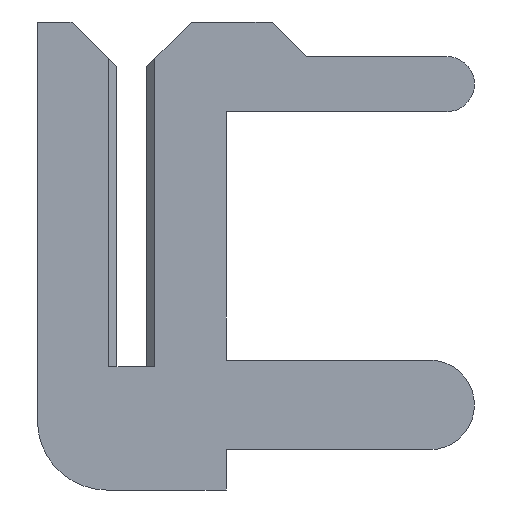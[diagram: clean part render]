
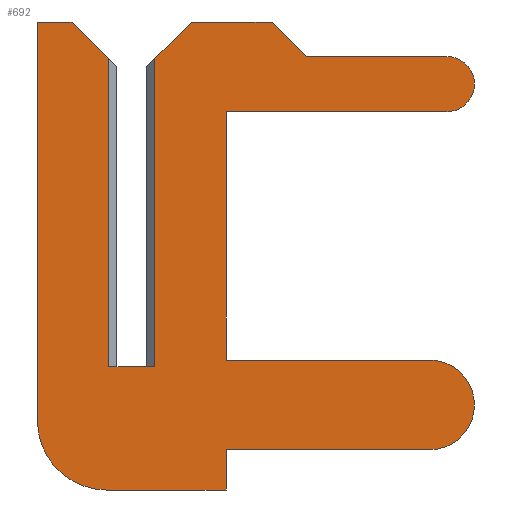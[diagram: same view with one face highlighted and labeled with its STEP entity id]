
A CAD part, left-side view. The second image highlights one B-rep face of the part: STEP entity #692.
In plain terms, the highlighted planar face has unit normal (-1, 0, 0).
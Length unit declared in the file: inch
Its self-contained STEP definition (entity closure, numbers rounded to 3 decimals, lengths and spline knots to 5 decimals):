
#9 = VECTOR ( 'NONE', #65, 39.37008 ) ;
#14 = DIRECTION ( 'NONE',  ( 0., 0., 1. ) ) ;
#15 = CARTESIAN_POINT ( 'NONE',  ( -0.01, -0.01, 0.134 ) ) ;
#26 = EDGE_CURVE ( 'NONE', #310, #512, #950, .T. ) ;
#29 = DIRECTION ( 'NONE',  ( 0., 0., -1. ) ) ;
#35 = CARTESIAN_POINT ( 'NONE',  ( -0.01, -0.076, 0.135 ) ) ;
#43 = VERTEX_POINT ( 'NONE', #170 ) ;
#44 = EDGE_CURVE ( 'NONE', #637, #543, #290, .T. ) ;
#54 = AXIS2_PLACEMENT_3D ( 'NONE', #1008, #584, #843 ) ;
#57 = CIRCLE ( 'NONE', #408, 0.0195 ) ;
#65 = DIRECTION ( 'NONE',  ( 0., 1., 0. ) ) ;
#67 = VERTEX_POINT ( 'NONE', #343 ) ;
#74 = AXIS2_PLACEMENT_3D ( 'NONE', #490, #242, #400 ) ;
#76 = VERTEX_POINT ( 'NONE', #622 ) ;
#88 = VECTOR ( 'NONE', #841, 39.37008 ) ;
#93 = CARTESIAN_POINT ( 'NONE',  ( -0.01, 0.026, 0.15 ) ) ;
#95 = CARTESIAN_POINT ( 'NONE',  ( -0.01, -0.1295, 0.003 ) ) ;
#98 = CARTESIAN_POINT ( 'NONE',  ( -0.01, 0.011, -0.0235 ) ) ;
#99 = LINE ( 'NONE', #196, #718 ) ;
#103 = EDGE_CURVE ( 'NONE', #399, #998, #57, .T. ) ;
#108 = CARTESIAN_POINT ( 'NONE',  ( -0.01, 0.041, 0.15 ) ) ;
#115 = VERTEX_POINT ( 'NONE', #700 ) ;
#123 = DIRECTION ( 'NONE',  ( 0., 0., 1. ) ) ;
#134 = EDGE_CURVE ( 'NONE', #356, #43, #860, .T. ) ;
#135 = LINE ( 'NONE', #108, #788 ) ;
#137 = DIRECTION ( 'NONE',  ( 0., 0., -1. ) ) ;
#145 = ORIENTED_EDGE ( 'NONE', *, *, #157, .F. ) ;
#155 = CARTESIAN_POINT ( 'NONE',  ( -0.01, -0.137, 0.135 ) ) ;
#157 = EDGE_CURVE ( 'NONE', #619, #431, #603, .T. ) ;
#170 = CARTESIAN_POINT ( 'NONE',  ( -0.01, -0.01, 0. ) ) ;
#180 = DIRECTION ( 'NONE',  ( 0., 1., 0. ) ) ;
#191 = LINE ( 'NONE', #1004, #9 ) ;
#195 = DIRECTION ( 'NONE',  ( 0., 1., 0. ) ) ;
#196 = CARTESIAN_POINT ( 'NONE',  ( -0.01, 0.01, -0.0235 ) ) ;
#198 = EDGE_LOOP ( 'NONE', ( #536, #684, #550, #1042, #621, #262, #651, #298, #620, #1079, #559, #703, #541, #442, #145, #604, #933, #417, #813 ) ) ;
#203 = CARTESIAN_POINT ( 'NONE',  ( -0.01, -0.076, 0.135 ) ) ;
#212 = CARTESIAN_POINT ( 'NONE',  ( -0.01, -0.0065, 0.1305 ) ) ;
#214 = DIRECTION ( 'NONE',  ( 0., -0.707, 0.707 ) ) ;
#221 = CARTESIAN_POINT ( 'NONE',  ( -0.01, 0.01, 0. ) ) ;
#229 = CARTESIAN_POINT ( 'NONE',  ( -0.01, -0.137, 0.135 ) ) ;
#235 = VECTOR ( 'NONE', #214, 39.37008 ) ;
#242 = DIRECTION ( 'NONE',  ( 1., 0., 0. ) ) ;
#253 = LINE ( 'NONE', #629, #313 ) ;
#257 = AXIS2_PLACEMENT_3D ( 'NONE', #98, #268, #1021 ) ;
#262 = ORIENTED_EDGE ( 'NONE', *, *, #44, .F. ) ;
#264 = EDGE_CURVE ( 'NONE', #800, #344, #485, .T. ) ;
#268 = DIRECTION ( 'NONE',  ( 1., 0., 0. ) ) ;
#270 = DIRECTION ( 'NONE',  ( 0., -1., 0. ) ) ;
#276 = EDGE_CURVE ( 'NONE', #831, #800, #565, .T. ) ;
#286 = VECTOR ( 'NONE', #270, 39.37008 ) ;
#290 = LINE ( 'NONE', #93, #376 ) ;
#294 = EDGE_CURVE ( 'NONE', #76, #558, #539, .T. ) ;
#298 = ORIENTED_EDGE ( 'NONE', *, *, #26, .F. ) ;
#310 = VERTEX_POINT ( 'NONE', #726 ) ;
#311 = VECTOR ( 'NONE', #1055, 39.37008 ) ;
#313 = VECTOR ( 'NONE', #137, 39.37008 ) ;
#314 = CARTESIAN_POINT ( 'NONE',  ( -0.01, 0.041, -0.0235 ) ) ;
#327 = VECTOR ( 'NONE', #875, 39.37008 ) ;
#337 = LINE ( 'NONE', #95, #286 ) ;
#339 = LINE ( 'NONE', #527, #434 ) ;
#343 = CARTESIAN_POINT ( 'NONE',  ( -0.01, 0.01, 0.134 ) ) ;
#344 = VERTEX_POINT ( 'NONE', #542 ) ;
#355 = DIRECTION ( 'NONE',  ( 1., 0., 0. ) ) ;
#356 = VERTEX_POINT ( 'NONE', #221 ) ;
#357 = CARTESIAN_POINT ( 'NONE',  ( -0.01, -0.041, -0.036 ) ) ;
#361 = VECTOR ( 'NONE', #466, 39.37008 ) ;
#371 = DIRECTION ( 'NONE',  ( 0., 0., -1. ) ) ;
#376 = VECTOR ( 'NONE', #520, 39.37008 ) ;
#377 = CARTESIAN_POINT ( 'NONE',  ( -0.01, -0.041, -0.0535 ) ) ;
#383 = EDGE_CURVE ( 'NONE', #431, #115, #253, .T. ) ;
#391 = LINE ( 'NONE', #155, #88 ) ;
#394 = CARTESIAN_POINT ( 'NONE',  ( -0.01, -0.041, -0.0535 ) ) ;
#399 = VERTEX_POINT ( 'NONE', #548 ) ;
#400 = DIRECTION ( 'NONE',  ( 0., 0., 1. ) ) ;
#408 = AXIS2_PLACEMENT_3D ( 'NONE', #712, #355, #529 ) ;
#413 = PLANE ( 'NONE',  #54 ) ;
#417 = ORIENTED_EDGE ( 'NONE', *, *, #922, .F. ) ;
#424 = CIRCLE ( 'NONE', #74, 0.012 ) ;
#431 = VERTEX_POINT ( 'NONE', #1071 ) ;
#434 = VECTOR ( 'NONE', #29, 39.37008 ) ;
#441 = CARTESIAN_POINT ( 'NONE',  ( -0.01, -0.026, 0.15 ) ) ;
#442 = ORIENTED_EDGE ( 'NONE', *, *, #383, .F. ) ;
#450 = CARTESIAN_POINT ( 'NONE',  ( -0.01, 0.0065, 0. ) ) ;
#457 = VECTOR ( 'NONE', #195, 39.37008 ) ;
#466 = DIRECTION ( 'NONE',  ( 0., -1., 0. ) ) ;
#485 = LINE ( 'NONE', #981, #361 ) ;
#490 = CARTESIAN_POINT ( 'NONE',  ( -0.01, -0.137, 0.123 ) ) ;
#498 = LINE ( 'NONE', #357, #870 ) ;
#501 = EDGE_CURVE ( 'NONE', #558, #310, #191, .T. ) ;
#512 = VERTEX_POINT ( 'NONE', #314 ) ;
#520 = DIRECTION ( 'NONE',  ( 0., -1., 0. ) ) ;
#527 = CARTESIAN_POINT ( 'NONE',  ( -0.01, -0.01, 0.15 ) ) ;
#529 = DIRECTION ( 'NONE',  ( 0., 0., 1. ) ) ;
#536 = ORIENTED_EDGE ( 'NONE', *, *, #276, .F. ) ;
#539 = LINE ( 'NONE', #377, #872 ) ;
#541 = ORIENTED_EDGE ( 'NONE', *, *, #807, .F. ) ;
#542 = CARTESIAN_POINT ( 'NONE',  ( -0.01, -0.061, 0.15 ) ) ;
#543 = VERTEX_POINT ( 'NONE', #999 ) ;
#548 = CARTESIAN_POINT ( 'NONE',  ( -0.01, -0.1295, 0.003 ) ) ;
#550 = ORIENTED_EDGE ( 'NONE', *, *, #134, .F. ) ;
#555 = EDGE_CURVE ( 'NONE', #1062, #619, #424, .T. ) ;
#558 = VERTEX_POINT ( 'NONE', #394 ) ;
#559 = ORIENTED_EDGE ( 'NONE', *, *, #829, .F. ) ;
#563 = FACE_OUTER_BOUND ( 'NONE', #198, .T. ) ;
#565 = LINE ( 'NONE', #212, #235 ) ;
#575 = LINE ( 'NONE', #944, #327 ) ;
#584 = DIRECTION ( 'NONE',  ( -1., 0., 0. ) ) ;
#585 = CARTESIAN_POINT ( 'NONE',  ( -0.01, 0.041, 0.15 ) ) ;
#597 = EDGE_CURVE ( 'NONE', #900, #1062, #391, .T. ) ;
#603 = LINE ( 'NONE', #873, #457 ) ;
#604 = ORIENTED_EDGE ( 'NONE', *, *, #555, .F. ) ;
#611 = LINE ( 'NONE', #203, #311 ) ;
#617 = DIRECTION ( 'NONE',  ( 0., -1., 0. ) ) ;
#619 = VERTEX_POINT ( 'NONE', #750 ) ;
#620 = ORIENTED_EDGE ( 'NONE', *, *, #501, .F. ) ;
#621 = ORIENTED_EDGE ( 'NONE', *, *, #767, .F. ) ;
#622 = CARTESIAN_POINT ( 'NONE',  ( -0.01, -0.041, -0.036 ) ) ;
#629 = CARTESIAN_POINT ( 'NONE',  ( -0.01, -0.041, 0.003 ) ) ;
#637 = VERTEX_POINT ( 'NONE', #585 ) ;
#651 = ORIENTED_EDGE ( 'NONE', *, *, #724, .F. ) ;
#655 = CARTESIAN_POINT ( 'NONE',  ( -0.01, -0.1295, -0.036 ) ) ;
#684 = ORIENTED_EDGE ( 'NONE', *, *, #710, .T. ) ;
#692 = ADVANCED_FACE ( 'NONE', ( #563 ), #413, .T. ) ;
#700 = CARTESIAN_POINT ( 'NONE',  ( -0.01, -0.041, 0.003 ) ) ;
#703 = ORIENTED_EDGE ( 'NONE', *, *, #103, .F. ) ;
#710 = EDGE_CURVE ( 'NONE', #831, #43, #339, .T. ) ;
#712 = CARTESIAN_POINT ( 'NONE',  ( -0.01, -0.1295, -0.0165 ) ) ;
#718 = VECTOR ( 'NONE', #123, 39.37008 ) ;
#724 = EDGE_CURVE ( 'NONE', #512, #637, #135, .T. ) ;
#726 = CARTESIAN_POINT ( 'NONE',  ( -0.01, 0.011, -0.0535 ) ) ;
#750 = CARTESIAN_POINT ( 'NONE',  ( -0.01, -0.137, 0.111 ) ) ;
#767 = EDGE_CURVE ( 'NONE', #543, #67, #575, .T. ) ;
#788 = VECTOR ( 'NONE', #14, 39.37008 ) ;
#800 = VERTEX_POINT ( 'NONE', #441 ) ;
#807 = EDGE_CURVE ( 'NONE', #115, #399, #337, .T. ) ;
#813 = ORIENTED_EDGE ( 'NONE', *, *, #264, .F. ) ;
#829 = EDGE_CURVE ( 'NONE', #998, #76, #498, .T. ) ;
#831 = VERTEX_POINT ( 'NONE', #15 ) ;
#841 = DIRECTION ( 'NONE',  ( 0., -1., 0. ) ) ;
#843 = DIRECTION ( 'NONE',  ( 0., 0., 1. ) ) ;
#860 = LINE ( 'NONE', #450, #1020 ) ;
#870 = VECTOR ( 'NONE', #180, 39.37008 ) ;
#872 = VECTOR ( 'NONE', #371, 39.37008 ) ;
#873 = CARTESIAN_POINT ( 'NONE',  ( -0.01, -0.041, 0.111 ) ) ;
#875 = DIRECTION ( 'NONE',  ( 0., -0.707, -0.707 ) ) ;
#900 = VERTEX_POINT ( 'NONE', #35 ) ;
#922 = EDGE_CURVE ( 'NONE', #344, #900, #611, .T. ) ;
#933 = ORIENTED_EDGE ( 'NONE', *, *, #597, .F. ) ;
#944 = CARTESIAN_POINT ( 'NONE',  ( -0.01, 0.0065, 0.1305 ) ) ;
#950 = CIRCLE ( 'NONE', #257, 0.03 ) ;
#956 = EDGE_CURVE ( 'NONE', #356, #67, #99, .T. ) ;
#981 = CARTESIAN_POINT ( 'NONE',  ( -0.01, -0.026, 0.15 ) ) ;
#998 = VERTEX_POINT ( 'NONE', #655 ) ;
#999 = CARTESIAN_POINT ( 'NONE',  ( -0.01, 0.026, 0.15 ) ) ;
#1004 = CARTESIAN_POINT ( 'NONE',  ( -0.01, 0.011, -0.0535 ) ) ;
#1008 = CARTESIAN_POINT ( 'NONE',  ( -0.01, 0.011, -0.0235 ) ) ;
#1020 = VECTOR ( 'NONE', #617, 39.37008 ) ;
#1021 = DIRECTION ( 'NONE',  ( 0., 0., 1. ) ) ;
#1042 = ORIENTED_EDGE ( 'NONE', *, *, #956, .T. ) ;
#1055 = DIRECTION ( 'NONE',  ( 0., -0.707, -0.707 ) ) ;
#1062 = VERTEX_POINT ( 'NONE', #229 ) ;
#1071 = CARTESIAN_POINT ( 'NONE',  ( -0.01, -0.041, 0.111 ) ) ;
#1079 = ORIENTED_EDGE ( 'NONE', *, *, #294, .F. ) ;
